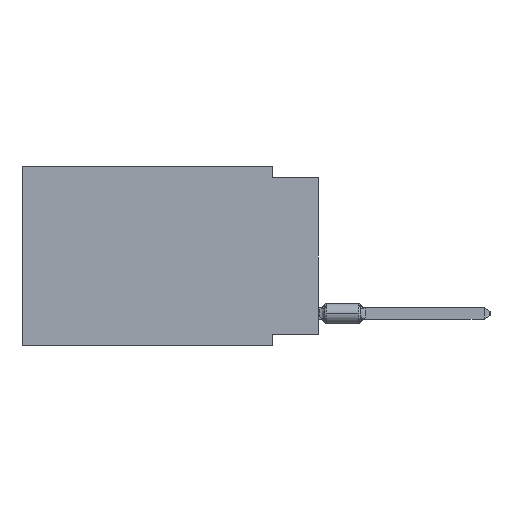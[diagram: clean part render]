
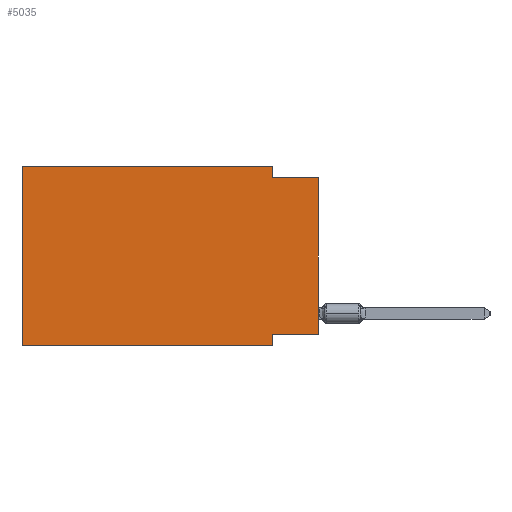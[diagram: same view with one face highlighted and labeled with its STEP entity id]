
A CAD part, left-side view. The second image highlights one B-rep face of the part: STEP entity #5035.
In plain terms, the highlighted planar face has unit normal (-1, 0, 0).
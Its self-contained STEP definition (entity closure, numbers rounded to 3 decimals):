
#414 = VERTEX_POINT ( 'NONE', #16658 ) ;
#1078 = ORIENTED_EDGE ( 'NONE', *, *, #10736, .F. ) ;
#2833 = DIRECTION ( 'NONE',  ( 0., 0., 1. ) ) ;
#3113 = CARTESIAN_POINT ( 'NONE',  ( 0., 2.54, 0. ) ) ;
#3606 = EDGE_CURVE ( 'NONE', #21666, #9722, #12584, .T. ) ;
#3899 = EDGE_CURVE ( 'NONE', #9722, #12007, #25061, .T. ) ;
#4102 = EDGE_CURVE ( 'NONE', #23147, #12941, #10966, .T. ) ;
#4375 = VECTOR ( 'NONE', #27152, 1000. ) ;
#5035 = ADVANCED_FACE ( 'NONE', ( #17464 ), #13093, .F. ) ;
#5238 = VERTEX_POINT ( 'NONE', #20274 ) ;
#5270 = VECTOR ( 'NONE', #16678, 1000. ) ;
#6082 = CARTESIAN_POINT ( 'NONE',  ( 0., 0., -9.271 ) ) ;
#6415 = VECTOR ( 'NONE', #16437, 1000. ) ;
#7114 = AXIS2_PLACEMENT_3D ( 'NONE', #12959, #23521, #10427 ) ;
#7572 = ORIENTED_EDGE ( 'NONE', *, *, #3606, .F. ) ;
#7725 = EDGE_CURVE ( 'NONE', #23011, #23147, #24389, .T. ) ;
#8574 = VECTOR ( 'NONE', #13843, 1000. ) ;
#8606 = CARTESIAN_POINT ( 'NONE',  ( 0., 2.54, -9.271 ) ) ;
#8840 = DIRECTION ( 'NONE',  ( 0., 0., -1. ) ) ;
#9722 = VERTEX_POINT ( 'NONE', #18627 ) ;
#10152 = ORIENTED_EDGE ( 'NONE', *, *, #7725, .F. ) ;
#10427 = DIRECTION ( 'NONE',  ( 0., 0., -1. ) ) ;
#10736 = EDGE_CURVE ( 'NONE', #414, #21666, #20934, .T. ) ;
#10966 = LINE ( 'NONE', #21805, #14302 ) ;
#11043 = CARTESIAN_POINT ( 'NONE',  ( 0., 0., 0. ) ) ;
#11281 = ORIENTED_EDGE ( 'NONE', *, *, #18851, .T. ) ;
#12007 = VERTEX_POINT ( 'NONE', #23137 ) ;
#12082 = CARTESIAN_POINT ( 'NONE',  ( 0., 16.383, -9.906 ) ) ;
#12584 = LINE ( 'NONE', #27757, #5270 ) ;
#12941 = VERTEX_POINT ( 'NONE', #21534 ) ;
#12959 = CARTESIAN_POINT ( 'NONE',  ( 0., 16.383, 0. ) ) ;
#13093 = PLANE ( 'NONE',  #7114 ) ;
#13843 = DIRECTION ( 'NONE',  ( 0., 1., 0. ) ) ;
#14062 = ORIENTED_EDGE ( 'NONE', *, *, #16313, .T. ) ;
#14302 = VECTOR ( 'NONE', #8840, 1000. ) ;
#16313 = EDGE_CURVE ( 'NONE', #23011, #12007, #22146, .T. ) ;
#16437 = DIRECTION ( 'NONE',  ( 0., -1., 0. ) ) ;
#16523 = CARTESIAN_POINT ( 'NONE',  ( 0., 16.383, 0. ) ) ;
#16658 = CARTESIAN_POINT ( 'NONE',  ( 0., 16.383, 0. ) ) ;
#16678 = DIRECTION ( 'NONE',  ( 0., 0., -1. ) ) ;
#17464 = FACE_OUTER_BOUND ( 'NONE', #20115, .T. ) ;
#17637 = CARTESIAN_POINT ( 'NONE',  ( 0., 0., -9.271 ) ) ;
#18627 = CARTESIAN_POINT ( 'NONE',  ( 0., 2.54, -0.635 ) ) ;
#18695 = DIRECTION ( 'NONE',  ( 0., -1., 0. ) ) ;
#18851 = EDGE_CURVE ( 'NONE', #5238, #12941, #23041, .T. ) ;
#18992 = CARTESIAN_POINT ( 'NONE',  ( 0., 0., -0.635 ) ) ;
#19105 = VECTOR ( 'NONE', #2833, 1000. ) ;
#19458 = ORIENTED_EDGE ( 'NONE', *, *, #20836, .F. ) ;
#20115 = EDGE_LOOP ( 'NONE', ( #14062, #24033, #7572, #1078, #19458, #11281, #21589, #10152 ) ) ;
#20274 = CARTESIAN_POINT ( 'NONE',  ( 0., 16.383, -9.906 ) ) ;
#20836 = EDGE_CURVE ( 'NONE', #5238, #414, #27197, .T. ) ;
#20934 = LINE ( 'NONE', #22764, #6415 ) ;
#21534 = CARTESIAN_POINT ( 'NONE',  ( 0., 2.54, -9.906 ) ) ;
#21589 = ORIENTED_EDGE ( 'NONE', *, *, #4102, .F. ) ;
#21666 = VERTEX_POINT ( 'NONE', #3113 ) ;
#21805 = CARTESIAN_POINT ( 'NONE',  ( 0., 2.54, -9.906 ) ) ;
#22146 = LINE ( 'NONE', #11043, #19105 ) ;
#22764 = CARTESIAN_POINT ( 'NONE',  ( 0., 16.383, 0. ) ) ;
#23011 = VERTEX_POINT ( 'NONE', #6082 ) ;
#23041 = LINE ( 'NONE', #12082, #26751 ) ;
#23137 = CARTESIAN_POINT ( 'NONE',  ( 0., 0., -0.635 ) ) ;
#23147 = VERTEX_POINT ( 'NONE', #8606 ) ;
#23521 = DIRECTION ( 'NONE',  ( 1., 0., 0. ) ) ;
#24033 = ORIENTED_EDGE ( 'NONE', *, *, #3899, .F. ) ;
#24389 = LINE ( 'NONE', #17637, #8574 ) ;
#24803 = VECTOR ( 'NONE', #25100, 1000. ) ;
#25061 = LINE ( 'NONE', #18992, #4375 ) ;
#25100 = DIRECTION ( 'NONE',  ( 0., 0., 1. ) ) ;
#26751 = VECTOR ( 'NONE', #18695, 1000. ) ;
#27152 = DIRECTION ( 'NONE',  ( 0., -1., 0. ) ) ;
#27197 = LINE ( 'NONE', #16523, #24803 ) ;
#27757 = CARTESIAN_POINT ( 'NONE',  ( 0., 2.54, 0. ) ) ;
